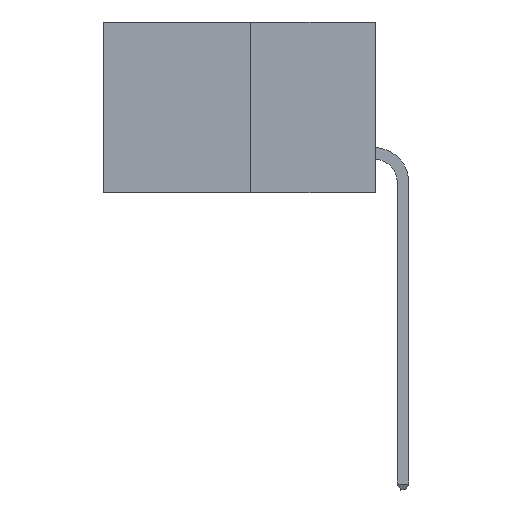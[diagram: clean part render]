
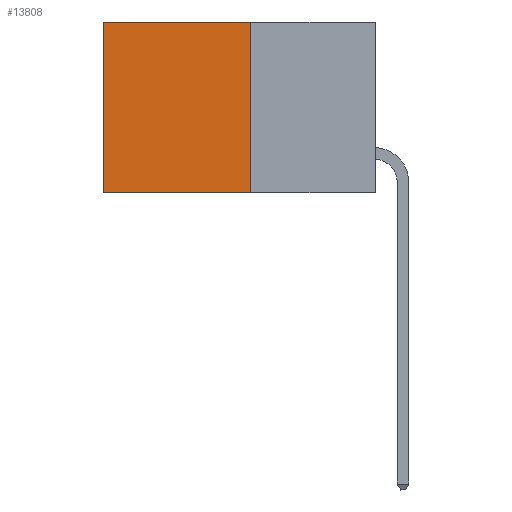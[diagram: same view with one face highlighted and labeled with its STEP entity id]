
A CAD part, left-side view. The second image highlights one B-rep face of the part: STEP entity #13808.
In plain terms, the highlighted planar face has unit normal (-1, 0, 0).
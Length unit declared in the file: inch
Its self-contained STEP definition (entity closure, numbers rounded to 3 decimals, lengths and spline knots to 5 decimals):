
#1108 = VECTOR ( 'NONE', #18811, 39.37008 ) ;
#1198 = CARTESIAN_POINT ( 'NONE',  ( 0.277, 0.59, -0.37 ) ) ;
#1258 = CARTESIAN_POINT ( 'NONE',  ( 0.277, 0.27, 0. ) ) ;
#1416 = VECTOR ( 'NONE', #2398, 39.37008 ) ;
#1638 = VECTOR ( 'NONE', #10854, 39.37008 ) ;
#2398 = DIRECTION ( 'NONE',  ( 0., 1., 0. ) ) ;
#2490 = CARTESIAN_POINT ( 'NONE',  ( 0.277, 0.27, 0. ) ) ;
#3430 = LINE ( 'NONE', #6911, #7199 ) ;
#4486 = PLANE ( 'NONE',  #15015 ) ;
#4529 = EDGE_CURVE ( 'NONE', #5627, #9237, #9722, .T. ) ;
#5627 = VERTEX_POINT ( 'NONE', #18627 ) ;
#5775 = VERTEX_POINT ( 'NONE', #17461 ) ;
#6142 = DIRECTION ( 'NONE',  ( 1., 0., 0. ) ) ;
#6780 = EDGE_LOOP ( 'NONE', ( #17308, #16376, #16934, #16077 ) ) ;
#6911 = CARTESIAN_POINT ( 'NONE',  ( 0.277, 0.27, -0.37 ) ) ;
#7199 = VECTOR ( 'NONE', #14907, 39.37008 ) ;
#9237 = VERTEX_POINT ( 'NONE', #1198 ) ;
#9712 = LINE ( 'NONE', #17230, #1108 ) ;
#9722 = LINE ( 'NONE', #12399, #1638 ) ;
#10008 = LINE ( 'NONE', #2490, #1416 ) ;
#10107 = EDGE_CURVE ( 'NONE', #19810, #5775, #10008, .T. ) ;
#10826 = EDGE_CURVE ( 'NONE', #19810, #5627, #3430, .T. ) ;
#10854 = DIRECTION ( 'NONE',  ( 0., 1., 0. ) ) ;
#12399 = CARTESIAN_POINT ( 'NONE',  ( 0.277, 0.27, -0.37 ) ) ;
#13808 = ADVANCED_FACE ( 'NONE', ( #18354 ), #4486, .F. ) ;
#14146 = CARTESIAN_POINT ( 'NONE',  ( 0.277, 0.27, -0.37 ) ) ;
#14907 = DIRECTION ( 'NONE',  ( 0., 0., -1. ) ) ;
#15015 = AXIS2_PLACEMENT_3D ( 'NONE', #14146, #6142, #17361 ) ;
#16077 = ORIENTED_EDGE ( 'NONE', *, *, #10107, .T. ) ;
#16376 = ORIENTED_EDGE ( 'NONE', *, *, #4529, .F. ) ;
#16934 = ORIENTED_EDGE ( 'NONE', *, *, #10826, .F. ) ;
#17230 = CARTESIAN_POINT ( 'NONE',  ( 0.277, 0.59, -0.37 ) ) ;
#17308 = ORIENTED_EDGE ( 'NONE', *, *, #19743, .T. ) ;
#17361 = DIRECTION ( 'NONE',  ( 0., 0., -1. ) ) ;
#17461 = CARTESIAN_POINT ( 'NONE',  ( 0.277, 0.59, 0. ) ) ;
#18354 = FACE_OUTER_BOUND ( 'NONE', #6780, .T. ) ;
#18627 = CARTESIAN_POINT ( 'NONE',  ( 0.277, 0.27, -0.37 ) ) ;
#18811 = DIRECTION ( 'NONE',  ( 0., 0., -1. ) ) ;
#19743 = EDGE_CURVE ( 'NONE', #5775, #9237, #9712, .T. ) ;
#19810 = VERTEX_POINT ( 'NONE', #1258 ) ;
